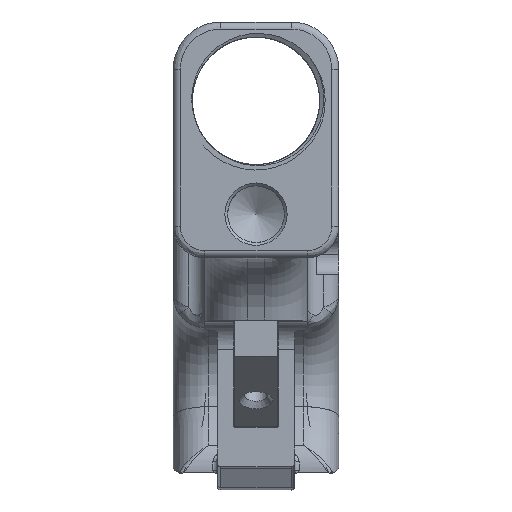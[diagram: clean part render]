
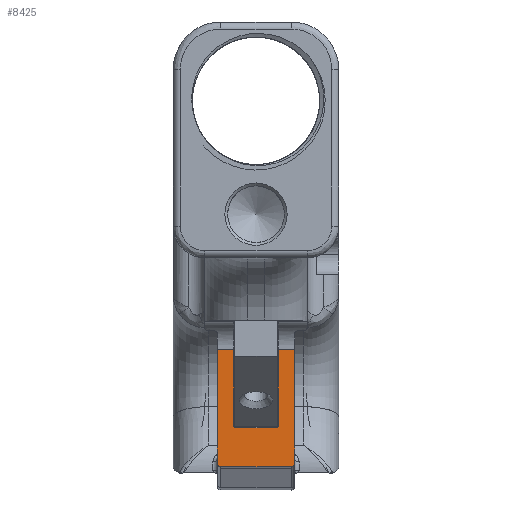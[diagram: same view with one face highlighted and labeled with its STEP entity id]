
A CAD part, left-side view. The second image highlights one B-rep face of the part: STEP entity #8425.
In plain terms, the highlighted planar face has unit normal (-1, 0, 0).
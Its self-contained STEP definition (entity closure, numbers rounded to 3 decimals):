
#106 = CARTESIAN_POINT ( 'NONE',  ( 32.64, 118.429, 97.414 ) ) ;
#465 = ORIENTED_EDGE ( 'NONE', *, *, #16558, .F. ) ;
#625 = VECTOR ( 'NONE', #31808, 1000. ) ;
#747 = EDGE_CURVE ( 'NONE', #26890, #19045, #22636, .T. ) ;
#836 = EDGE_CURVE ( 'NONE', #16138, #22441, #29607, .T. ) ;
#878 = LINE ( 'NONE', #23214, #35768 ) ;
#1009 = EDGE_CURVE ( 'NONE', #12509, #34453, #16504, .T. ) ;
#1268 = CARTESIAN_POINT ( 'NONE',  ( 32.64, 119.223, 123.678 ) ) ;
#4245 = CARTESIAN_POINT ( 'NONE',  ( 32.64, 119.223, 157.091 ) ) ;
#4269 = DIRECTION ( 'NONE',  ( 0., 0., -1. ) ) ;
#4698 = CARTESIAN_POINT ( 'NONE',  ( 32.64, 101.925, 98.227 ) ) ;
#4942 = DIRECTION ( 'NONE',  ( -1., 0., 0. ) ) ;
#5628 = DIRECTION ( 'NONE',  ( 0., 0., 1. ) ) ;
#5725 = VECTOR ( 'NONE', #24909, 1000. ) ;
#6217 = ORIENTED_EDGE ( 'NONE', *, *, #16939, .F. ) ;
#6468 = CARTESIAN_POINT ( 'NONE',  ( 32.64, 115.591, 106.66 ) ) ;
#6624 = VERTEX_POINT ( 'NONE', #30437 ) ;
#6682 = CARTESIAN_POINT ( 'NONE',  ( 32.64, 102.719, 97.414 ) ) ;
#6727 = ORIENTED_EDGE ( 'NONE', *, *, #33086, .F. ) ;
#7197 = PLANE ( 'NONE',  #30729 ) ;
#8425 = ADVANCED_FACE ( 'NONE', ( #8946 ), #7197, .F. ) ;
#8504 = ORIENTED_EDGE ( 'NONE', *, *, #747, .F. ) ;
#8569 = CARTESIAN_POINT ( 'NONE',  ( 32.64, 118.894, 97.414 ) ) ;
#8793 = EDGE_CURVE ( 'NONE', #22441, #6624, #878, .T. ) ;
#8822 = CARTESIAN_POINT ( 'NONE',  ( 32.64, 102.719, 97.414 ) ) ;
#8939 = ORIENTED_EDGE ( 'NONE', *, *, #21432, .F. ) ;
#8945 = CARTESIAN_POINT ( 'NONE',  ( 32.64, 101.925, 97.751 ) ) ;
#8946 = FACE_OUTER_BOUND ( 'NONE', #18827, .T. ) ;
#9825 = DIRECTION ( 'NONE',  ( 0., -1., 0. ) ) ;
#10135 = AXIS2_PLACEMENT_3D ( 'NONE', #22516, #4942, #25451 ) ;
#10266 = LINE ( 'NONE', #1268, #25883 ) ;
#11487 = DIRECTION ( 'NONE',  ( 0., -1., 0. ) ) ;
#11637 = CARTESIAN_POINT ( 'NONE',  ( 32.64, 102.254, 97.414 ) ) ;
#12144 = LINE ( 'NONE', #24777, #35074 ) ;
#12509 = VERTEX_POINT ( 'NONE', #4698 ) ;
#12566 = ORIENTED_EDGE ( 'NONE', *, *, #8793, .F. ) ;
#13086 = DIRECTION ( 'NONE',  ( 1., 0., 0. ) ) ;
#13350 = VERTEX_POINT ( 'NONE', #24519 ) ;
#13453 = EDGE_CURVE ( 'NONE', #22515, #19045, #12144, .T. ) ;
#13479 = AXIS2_PLACEMENT_3D ( 'NONE', #13880, #14170, #14340 ) ;
#13853 = ORIENTED_EDGE ( 'NONE', *, *, #836, .F. ) ;
#13880 = CARTESIAN_POINT ( 'NONE',  ( 32.64, 106.066, 106.66 ) ) ;
#14170 = DIRECTION ( 'NONE',  ( -1., 0., 0. ) ) ;
#14192 = CARTESIAN_POINT ( 'NONE',  ( 32.64, 115.591, 157.091 ) ) ;
#14340 = DIRECTION ( 'NONE',  ( 0., -1., 0. ) ) ;
#15596 = EDGE_CURVE ( 'NONE', #37333, #21198, #26753, .T. ) ;
#16138 = VERTEX_POINT ( 'NONE', #21230 ) ;
#16297 = CARTESIAN_POINT ( 'NONE',  ( 32.64, 119.223, 97.414 ) ) ;
#16424 = VECTOR ( 'NONE', #25136, 1000. ) ;
#16504 =( BOUNDED_CURVE ( )  B_SPLINE_CURVE ( 3, ( #17551, #8945, #11637, #8822 ),
 .UNSPECIFIED., .F., .F. ) 
 B_SPLINE_CURVE_WITH_KNOTS ( ( 4, 4 ),
 ( 1.571, 3.142 ),
 .UNSPECIFIED. ) 
 CURVE ( )  GEOMETRIC_REPRESENTATION_ITEM ( )  RATIONAL_B_SPLINE_CURVE ( ( 1., 0.805, 0.805, 1. ) ) 
 REPRESENTATION_ITEM ( '' )  );
#16558 = EDGE_CURVE ( 'NONE', #21198, #30918, #37519, .T. ) ;
#16939 = EDGE_CURVE ( 'NONE', #6624, #13350, #27946, .T. ) ;
#17461 = CARTESIAN_POINT ( 'NONE',  ( 32.64, 119.223, 106.152 ) ) ;
#17551 = CARTESIAN_POINT ( 'NONE',  ( 32.64, 101.925, 98.227 ) ) ;
#18827 = EDGE_LOOP ( 'NONE', ( #32608, #6727, #27984, #8504, #24126, #34337, #19179, #6217, #12566, #13853, #8939, #465 ) ) ;
#19045 = VERTEX_POINT ( 'NONE', #20983 ) ;
#19179 = ORIENTED_EDGE ( 'NONE', *, *, #31805, .F. ) ;
#20269 = DIRECTION ( 'NONE',  ( 0., -1., 0. ) ) ;
#20983 = CARTESIAN_POINT ( 'NONE',  ( 32.64, 119.223, 98.227 ) ) ;
#21198 = VERTEX_POINT ( 'NONE', #6468 ) ;
#21230 = CARTESIAN_POINT ( 'NONE',  ( 32.64, 106.066, 106.152 ) ) ;
#21432 = EDGE_CURVE ( 'NONE', #30918, #16138, #23268, .T. ) ;
#21975 = CARTESIAN_POINT ( 'NONE',  ( 32.64, 101.925, 157.091 ) ) ;
#22441 = VERTEX_POINT ( 'NONE', #26750 ) ;
#22515 = VERTEX_POINT ( 'NONE', #32824 ) ;
#22516 = CARTESIAN_POINT ( 'NONE',  ( 32.64, 115.083, 106.66 ) ) ;
#22636 =( BOUNDED_CURVE ( )  B_SPLINE_CURVE ( 3, ( #24704, #8569, #35150, #24964 ),
 .UNSPECIFIED., .F., .T. ) 
 B_SPLINE_CURVE_WITH_KNOTS ( ( 4, 4 ),
 ( 0., 1.571 ),
 .UNSPECIFIED. ) 
 CURVE ( )  GEOMETRIC_REPRESENTATION_ITEM ( )  RATIONAL_B_SPLINE_CURVE ( ( 1., 0.805, 0.805, 1. ) ) 
 REPRESENTATION_ITEM ( '' )  );
#23214 = CARTESIAN_POINT ( 'NONE',  ( 32.64, 105.558, 157.091 ) ) ;
#23268 = LINE ( 'NONE', #17461, #30172 ) ;
#24126 = ORIENTED_EDGE ( 'NONE', *, *, #25240, .F. ) ;
#24519 = CARTESIAN_POINT ( 'NONE',  ( 32.64, 101.925, 123.678 ) ) ;
#24704 = CARTESIAN_POINT ( 'NONE',  ( 32.64, 118.429, 97.414 ) ) ;
#24777 = CARTESIAN_POINT ( 'NONE',  ( 32.64, 119.223, 157.091 ) ) ;
#24909 = DIRECTION ( 'NONE',  ( 0., 0., -1. ) ) ;
#24964 = CARTESIAN_POINT ( 'NONE',  ( 32.64, 119.223, 98.227 ) ) ;
#25136 = DIRECTION ( 'NONE',  ( 0., 1., 0. ) ) ;
#25240 = EDGE_CURVE ( 'NONE', #34453, #26890, #26042, .T. ) ;
#25451 = DIRECTION ( 'NONE',  ( 0., -1., 0. ) ) ;
#25513 = VECTOR ( 'NONE', #11487, 1000. ) ;
#25883 = VECTOR ( 'NONE', #9825, 1000. ) ;
#25904 = CARTESIAN_POINT ( 'NONE',  ( 32.64, 115.591, 123.678 ) ) ;
#26042 = LINE ( 'NONE', #16297, #16424 ) ;
#26750 = CARTESIAN_POINT ( 'NONE',  ( 32.64, 105.558, 106.66 ) ) ;
#26753 = LINE ( 'NONE', #14192, #625 ) ;
#26890 = VERTEX_POINT ( 'NONE', #106 ) ;
#27946 = LINE ( 'NONE', #32045, #25513 ) ;
#27984 = ORIENTED_EDGE ( 'NONE', *, *, #13453, .T. ) ;
#29134 = LINE ( 'NONE', #21975, #5725 ) ;
#29607 = CIRCLE ( 'NONE', #13479, 0.508 ) ;
#30172 = VECTOR ( 'NONE', #20269, 1000. ) ;
#30437 = CARTESIAN_POINT ( 'NONE',  ( 32.64, 105.558, 123.678 ) ) ;
#30729 = AXIS2_PLACEMENT_3D ( 'NONE', #4245, #13086, #33635 ) ;
#30918 = VERTEX_POINT ( 'NONE', #37662 ) ;
#31805 = EDGE_CURVE ( 'NONE', #13350, #12509, #29134, .T. ) ;
#31808 = DIRECTION ( 'NONE',  ( 0., 0., -1. ) ) ;
#32045 = CARTESIAN_POINT ( 'NONE',  ( 32.64, 119.223, 123.678 ) ) ;
#32608 = ORIENTED_EDGE ( 'NONE', *, *, #15596, .F. ) ;
#32824 = CARTESIAN_POINT ( 'NONE',  ( 32.64, 119.223, 123.678 ) ) ;
#33086 = EDGE_CURVE ( 'NONE', #22515, #37333, #10266, .T. ) ;
#33635 = DIRECTION ( 'NONE',  ( 0., 0., 1. ) ) ;
#34337 = ORIENTED_EDGE ( 'NONE', *, *, #1009, .F. ) ;
#34453 = VERTEX_POINT ( 'NONE', #6682 ) ;
#35074 = VECTOR ( 'NONE', #4269, 1000. ) ;
#35150 = CARTESIAN_POINT ( 'NONE',  ( 32.64, 119.223, 97.751 ) ) ;
#35768 = VECTOR ( 'NONE', #5628, 1000. ) ;
#37333 = VERTEX_POINT ( 'NONE', #25904 ) ;
#37519 = CIRCLE ( 'NONE', #10135, 0.508 ) ;
#37662 = CARTESIAN_POINT ( 'NONE',  ( 32.64, 115.083, 106.152 ) ) ;
